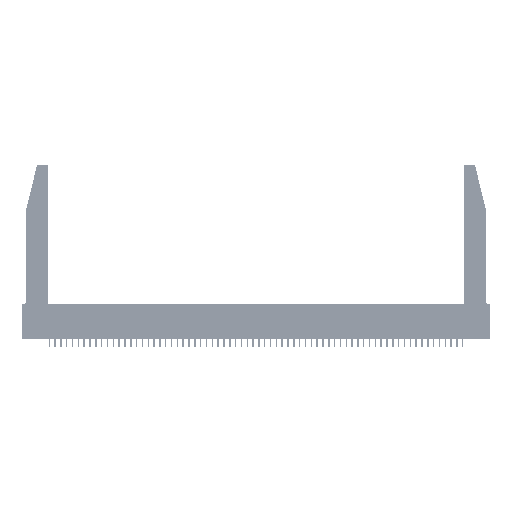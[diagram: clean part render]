
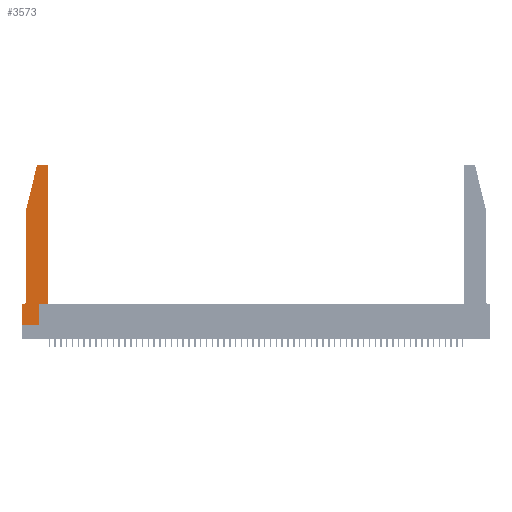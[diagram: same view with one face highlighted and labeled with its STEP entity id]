
A CAD part, top view. The second image highlights one B-rep face of the part: STEP entity #3573.
In plain terms, the highlighted planar face has unit normal (0, 0, 1).
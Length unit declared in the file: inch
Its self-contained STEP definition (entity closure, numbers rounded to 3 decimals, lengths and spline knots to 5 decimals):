
#401 = CARTESIAN_POINT ( 'NONE',  ( 0.4505, 0.35, 0.37 ) ) ;
#548 = CARTESIAN_POINT ( 'NONE',  ( 0.0055, 0.35, 0.37 ) ) ;
#2414 = DIRECTION ( 'NONE',  ( 1., 0., 0. ) ) ;
#3573 = ADVANCED_FACE ( 'NONE', ( #43926 ), #18157, .T. ) ;
#3658 = CARTESIAN_POINT ( 'NONE',  ( 0., 0.35, 0.37 ) ) ;
#3870 = LINE ( 'NONE', #51898, #49514 ) ;
#4118 = ORIENTED_EDGE ( 'NONE', *, *, #8206, .T. ) ;
#4309 = DIRECTION ( 'NONE',  ( 0., 0., 1. ) ) ;
#4856 = DIRECTION ( 'NONE',  ( 0., 1., 0. ) ) ;
#5092 = EDGE_CURVE ( 'NONE', #9610, #36006, #39616, .T. ) ;
#6567 = CARTESIAN_POINT ( 'NONE',  ( 0.0755, 0.42, 0.37 ) ) ;
#7088 = VERTEX_POINT ( 'NONE', #48413 ) ;
#7134 = ORIENTED_EDGE ( 'NONE', *, *, #26666, .T. ) ;
#7726 = ORIENTED_EDGE ( 'NONE', *, *, #14516, .T. ) ;
#7994 = CARTESIAN_POINT ( 'NONE',  ( 0.0755, 2., 0.37 ) ) ;
#8171 = LINE ( 'NONE', #7994, #17149 ) ;
#8206 = EDGE_CURVE ( 'NONE', #30334, #45720, #43394, .T. ) ;
#9396 = EDGE_CURVE ( 'NONE', #32045, #50507, #37634, .T. ) ;
#9483 = DIRECTION ( 'NONE',  ( 1., 0., 0. ) ) ;
#9610 = VERTEX_POINT ( 'NONE', #35480 ) ;
#11182 = CARTESIAN_POINT ( 'NONE',  ( 0., 0., 0.37 ) ) ;
#11349 = CARTESIAN_POINT ( 'NONE',  ( 0.4505, 0.35, 0.37 ) ) ;
#11808 = AXIS2_PLACEMENT_3D ( 'NONE', #29837, #38317, #39073 ) ;
#11830 = LINE ( 'NONE', #11349, #42202 ) ;
#12176 = CARTESIAN_POINT ( 'NONE',  ( 0., 0., 0.37 ) ) ;
#12277 = VERTEX_POINT ( 'NONE', #22445 ) ;
#12575 = ORIENTED_EDGE ( 'NONE', *, *, #9396, .T. ) ;
#12893 = ORIENTED_EDGE ( 'NONE', *, *, #5092, .T. ) ;
#13400 = ORIENTED_EDGE ( 'NONE', *, *, #16265, .T. ) ;
#13548 = ORIENTED_EDGE ( 'NONE', *, *, #37979, .T. ) ;
#14184 = ORIENTED_EDGE ( 'NONE', *, *, #21151, .T. ) ;
#14509 = AXIS2_PLACEMENT_3D ( 'NONE', #21894, #4309, #22289 ) ;
#14516 = EDGE_CURVE ( 'NONE', #36006, #7088, #49461, .T. ) ;
#14778 = VECTOR ( 'NONE', #2414, 39.37008 ) ;
#15234 = LINE ( 'NONE', #401, #37340 ) ;
#15607 = VECTOR ( 'NONE', #18203, 39.37008 ) ;
#16265 = EDGE_CURVE ( 'NONE', #12277, #18762, #29504, .T. ) ;
#16893 = EDGE_LOOP ( 'NONE', ( #21650, #4118, #38113, #54782, #12575, #7134, #14184, #12893, #7726, #13548, #20350, #13400 ) ) ;
#17149 = VECTOR ( 'NONE', #42952, 39.37008 ) ;
#17302 = CARTESIAN_POINT ( 'NONE',  ( 0.0755, 2., 0.37 ) ) ;
#18056 = VERTEX_POINT ( 'NONE', #17302 ) ;
#18157 = PLANE ( 'NONE',  #33597 ) ;
#18203 = DIRECTION ( 'NONE',  ( 0., 1., 0. ) ) ;
#18762 = VERTEX_POINT ( 'NONE', #45400 ) ;
#20350 = ORIENTED_EDGE ( 'NONE', *, *, #44296, .T. ) ;
#21052 = CARTESIAN_POINT ( 'NONE',  ( 0.25487, 2.72718, 0.37 ) ) ;
#21151 = EDGE_CURVE ( 'NONE', #52085, #9610, #34422, .T. ) ;
#21650 = ORIENTED_EDGE ( 'NONE', *, *, #27441, .T. ) ;
#21686 = LINE ( 'NONE', #36974, #37596 ) ;
#21838 = EDGE_CURVE ( 'NONE', #18056, #32045, #8171, .T. ) ;
#21894 = CARTESIAN_POINT ( 'NONE',  ( 0.284, 2.72, 0.37 ) ) ;
#21904 = AXIS2_PLACEMENT_3D ( 'NONE', #25268, #25450, #55796 ) ;
#22289 = DIRECTION ( 'NONE',  ( 1., 0., 0. ) ) ;
#22445 = CARTESIAN_POINT ( 'NONE',  ( 0.4505, 2.72, 0.37 ) ) ;
#22695 = VECTOR ( 'NONE', #29915, 39.37008 ) ;
#24374 = DIRECTION ( 'NONE',  ( -1., 0., 0. ) ) ;
#25268 = CARTESIAN_POINT ( 'NONE',  ( 0.0055, 0.42, 0.37 ) ) ;
#25450 = DIRECTION ( 'NONE',  ( 0., 0., -1. ) ) ;
#25605 = CARTESIAN_POINT ( 'NONE',  ( 0.2865, 0., 0.37 ) ) ;
#25899 = EDGE_CURVE ( 'NONE', #45720, #18056, #3870, .T. ) ;
#26666 = EDGE_CURVE ( 'NONE', #50507, #52085, #50798, .T. ) ;
#27441 = EDGE_CURVE ( 'NONE', #18762, #30334, #21686, .T. ) ;
#28671 = VECTOR ( 'NONE', #48416, 39.37008 ) ;
#28791 = CARTESIAN_POINT ( 'NONE',  ( 0.284, 2.75, 0.37 ) ) ;
#29504 = CIRCLE ( 'NONE', #11808, 0.03 ) ;
#29837 = CARTESIAN_POINT ( 'NONE',  ( 0.4205, 2.72, 0.37 ) ) ;
#29915 = DIRECTION ( 'NONE',  ( 0., -1., 0. ) ) ;
#30057 = DIRECTION ( 'NONE',  ( -0.239, -0.971, 0. ) ) ;
#30334 = VERTEX_POINT ( 'NONE', #28791 ) ;
#31492 = CARTESIAN_POINT ( 'NONE',  ( 0., 0.35, 0.37 ) ) ;
#32045 = VERTEX_POINT ( 'NONE', #6567 ) ;
#33597 = AXIS2_PLACEMENT_3D ( 'NONE', #31492, #35937, #9483 ) ;
#34422 = LINE ( 'NONE', #12176, #22695 ) ;
#34427 = CARTESIAN_POINT ( 'NONE',  ( 0.4505, 0.35, 0.37 ) ) ;
#35206 = CARTESIAN_POINT ( 'NONE',  ( 0.2865, 0.35, 0.37 ) ) ;
#35480 = CARTESIAN_POINT ( 'NONE',  ( 0., 0., 0.37 ) ) ;
#35937 = DIRECTION ( 'NONE',  ( 0., 0., 1. ) ) ;
#36006 = VERTEX_POINT ( 'NONE', #25605 ) ;
#36974 = CARTESIAN_POINT ( 'NONE',  ( 0.2605, 2.75, 0.37 ) ) ;
#37340 = VECTOR ( 'NONE', #4856, 39.37008 ) ;
#37596 = VECTOR ( 'NONE', #24374, 39.37008 ) ;
#37634 = CIRCLE ( 'NONE', #21904, 0.07 ) ;
#37979 = EDGE_CURVE ( 'NONE', #7088, #44025, #11830, .T. ) ;
#38113 = ORIENTED_EDGE ( 'NONE', *, *, #25899, .T. ) ;
#38317 = DIRECTION ( 'NONE',  ( 0., 0., 1. ) ) ;
#39073 = DIRECTION ( 'NONE',  ( 1., 0., 0. ) ) ;
#39616 = LINE ( 'NONE', #11182, #14778 ) ;
#42202 = VECTOR ( 'NONE', #55941, 39.37008 ) ;
#42952 = DIRECTION ( 'NONE',  ( 0., -1., 0. ) ) ;
#43394 = CIRCLE ( 'NONE', #14509, 0.03 ) ;
#43926 = FACE_OUTER_BOUND ( 'NONE', #16893, .T. ) ;
#44025 = VERTEX_POINT ( 'NONE', #34427 ) ;
#44296 = EDGE_CURVE ( 'NONE', #44025, #12277, #15234, .T. ) ;
#45400 = CARTESIAN_POINT ( 'NONE',  ( 0.4205, 2.75, 0.37 ) ) ;
#45720 = VERTEX_POINT ( 'NONE', #21052 ) ;
#48413 = CARTESIAN_POINT ( 'NONE',  ( 0.2865, 0.35, 0.37 ) ) ;
#48416 = DIRECTION ( 'NONE',  ( -1., 0., 0. ) ) ;
#49461 = LINE ( 'NONE', #35206, #15607 ) ;
#49514 = VECTOR ( 'NONE', #30057, 39.37008 ) ;
#50507 = VERTEX_POINT ( 'NONE', #548 ) ;
#50798 = LINE ( 'NONE', #52669, #28671 ) ;
#51898 = CARTESIAN_POINT ( 'NONE',  ( 0.0755, 2., 0.37 ) ) ;
#52085 = VERTEX_POINT ( 'NONE', #3658 ) ;
#52669 = CARTESIAN_POINT ( 'NONE',  ( 0.0755, 0.35, 0.37 ) ) ;
#54782 = ORIENTED_EDGE ( 'NONE', *, *, #21838, .T. ) ;
#55796 = DIRECTION ( 'NONE',  ( -1., 0., 0. ) ) ;
#55941 = DIRECTION ( 'NONE',  ( 1., 0., 0. ) ) ;
